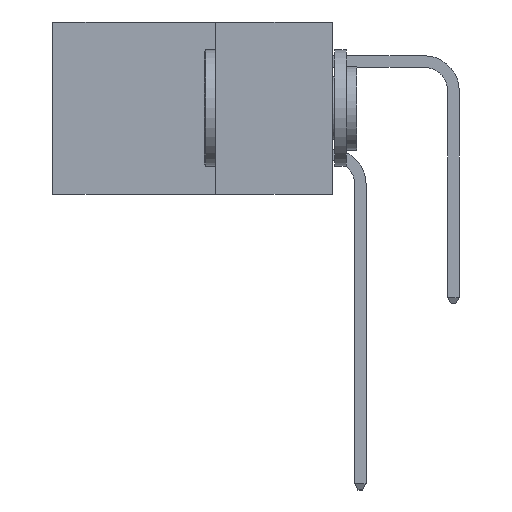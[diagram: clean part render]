
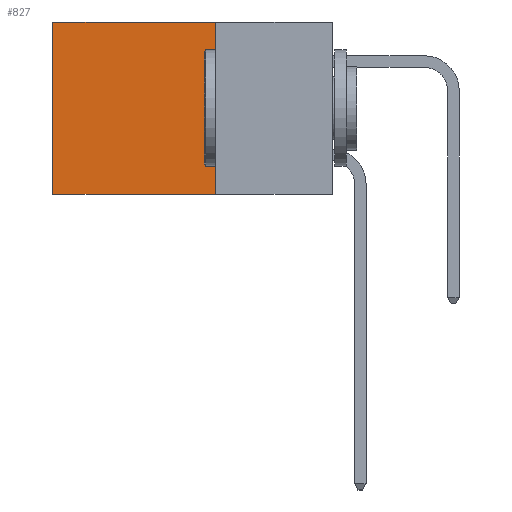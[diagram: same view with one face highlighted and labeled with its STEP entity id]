
A CAD part, left-side view. The second image highlights one B-rep face of the part: STEP entity #827.
In plain terms, the highlighted planar face has unit normal (-1, 0, 0).
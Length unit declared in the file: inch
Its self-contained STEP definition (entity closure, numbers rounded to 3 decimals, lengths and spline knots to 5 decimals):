
#770 = PLANE ( 'NONE',  #4252 ) ;
#827 = ADVANCED_FACE ( 'NONE', ( #15540 ), #770, .F. ) ;
#1311 = DIRECTION ( 'NONE',  ( 0., 1., 0. ) ) ;
#1608 = LINE ( 'NONE', #13264, #18548 ) ;
#2073 = DIRECTION ( 'NONE',  ( 0., 0., -1. ) ) ;
#3551 = VERTEX_POINT ( 'NONE', #3855 ) ;
#3741 = VECTOR ( 'NONE', #9956, 39.37008 ) ;
#3855 = CARTESIAN_POINT ( 'NONE',  ( 0.2615, 0.25, 0. ) ) ;
#4164 = VERTEX_POINT ( 'NONE', #11601 ) ;
#4252 = AXIS2_PLACEMENT_3D ( 'NONE', #10842, #6804, #2073 ) ;
#4340 = CARTESIAN_POINT ( 'NONE',  ( 0.2615, 0.25, -0.37 ) ) ;
#5318 = VERTEX_POINT ( 'NONE', #4340 ) ;
#6275 = CARTESIAN_POINT ( 'NONE',  ( 0.2615, 0.25, -0.37 ) ) ;
#6804 = DIRECTION ( 'NONE',  ( 1., 0., 0. ) ) ;
#8092 = CARTESIAN_POINT ( 'NONE',  ( 0.2615, 0.25, 0. ) ) ;
#8249 = LINE ( 'NONE', #6275, #19747 ) ;
#8428 = CARTESIAN_POINT ( 'NONE',  ( 0.2615, 0.6, 0. ) ) ;
#9956 = DIRECTION ( 'NONE',  ( 0., 0., -1. ) ) ;
#10035 = CARTESIAN_POINT ( 'NONE',  ( 0.2615, 0.6, -0.37 ) ) ;
#10842 = CARTESIAN_POINT ( 'NONE',  ( 0.2615, 0.25, -0.37 ) ) ;
#11601 = CARTESIAN_POINT ( 'NONE',  ( 0.2615, 0.6, -0.37 ) ) ;
#12521 = ORIENTED_EDGE ( 'NONE', *, *, #14447, .T. ) ;
#13264 = CARTESIAN_POINT ( 'NONE',  ( 0.2615, 0.25, -0.37 ) ) ;
#13560 = ORIENTED_EDGE ( 'NONE', *, *, #18756, .T. ) ;
#13999 = ORIENTED_EDGE ( 'NONE', *, *, #19344, .F. ) ;
#14447 = EDGE_CURVE ( 'NONE', #3551, #21261, #19507, .T. ) ;
#15089 = EDGE_CURVE ( 'NONE', #5318, #4164, #8249, .T. ) ;
#15540 = FACE_OUTER_BOUND ( 'NONE', #15970, .T. ) ;
#15970 = EDGE_LOOP ( 'NONE', ( #13560, #16581, #13999, #12521 ) ) ;
#16199 = DIRECTION ( 'NONE',  ( 0., 1., 0. ) ) ;
#16581 = ORIENTED_EDGE ( 'NONE', *, *, #15089, .F. ) ;
#18548 = VECTOR ( 'NONE', #19792, 39.37008 ) ;
#18756 = EDGE_CURVE ( 'NONE', #21261, #4164, #21143, .T. ) ;
#18987 = VECTOR ( 'NONE', #16199, 39.37008 ) ;
#19344 = EDGE_CURVE ( 'NONE', #3551, #5318, #1608, .T. ) ;
#19507 = LINE ( 'NONE', #8092, #18987 ) ;
#19747 = VECTOR ( 'NONE', #1311, 39.37008 ) ;
#19792 = DIRECTION ( 'NONE',  ( 0., 0., -1. ) ) ;
#21143 = LINE ( 'NONE', #10035, #3741 ) ;
#21261 = VERTEX_POINT ( 'NONE', #8428 ) ;
